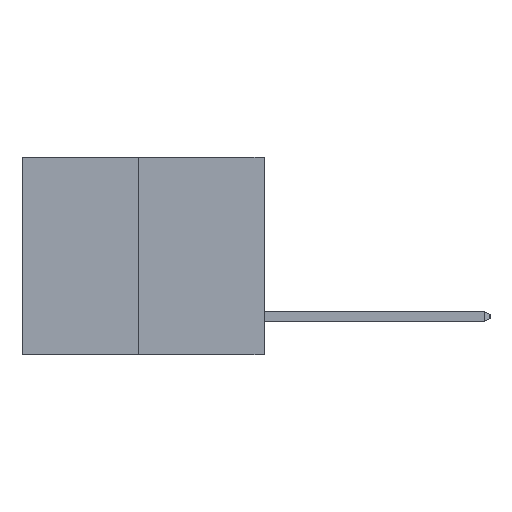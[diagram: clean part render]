
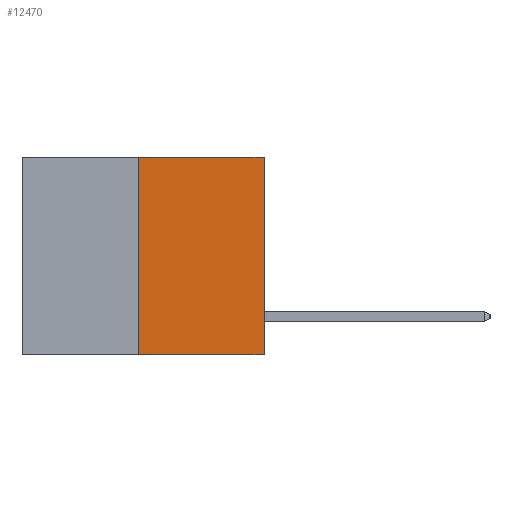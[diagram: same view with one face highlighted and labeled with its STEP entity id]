
A CAD part, left-side view. The second image highlights one B-rep face of the part: STEP entity #12470.
In plain terms, the highlighted planar face has unit normal (-1, 0, 0).
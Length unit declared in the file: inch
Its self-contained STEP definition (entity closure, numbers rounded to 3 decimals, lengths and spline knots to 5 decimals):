
#847 = ORIENTED_EDGE ( 'NONE', *, *, #9209, .F. ) ;
#1456 = DIRECTION ( 'NONE',  ( 0., 0., 1. ) ) ;
#1790 = PLANE ( 'NONE',  #20895 ) ;
#2164 = ORIENTED_EDGE ( 'NONE', *, *, #15549, .T. ) ;
#3511 = VERTEX_POINT ( 'NONE', #18823 ) ;
#3565 = DIRECTION ( 'NONE',  ( 0., 0., -1. ) ) ;
#3786 = DIRECTION ( 'NONE',  ( 1., 0., 0. ) ) ;
#4258 = EDGE_CURVE ( 'NONE', #3511, #21067, #6278, .T. ) ;
#5006 = LINE ( 'NONE', #19514, #7952 ) ;
#5191 = FACE_OUTER_BOUND ( 'NONE', #20338, .T. ) ;
#6278 = LINE ( 'NONE', #20141, #17500 ) ;
#6523 = LINE ( 'NONE', #18433, #20125 ) ;
#7952 = VECTOR ( 'NONE', #9261, 39.37008 ) ;
#8284 = DIRECTION ( 'NONE',  ( 0., 0., 1. ) ) ;
#9209 = EDGE_CURVE ( 'NONE', #15320, #20425, #6523, .T. ) ;
#9261 = DIRECTION ( 'NONE',  ( 0., -1., 0. ) ) ;
#9698 = CARTESIAN_POINT ( 'NONE',  ( 0., 0., 0. ) ) ;
#9887 = EDGE_CURVE ( 'NONE', #20425, #21067, #5006, .T. ) ;
#10288 = LINE ( 'NONE', #18601, #11376 ) ;
#11376 = VECTOR ( 'NONE', #18529, 39.37008 ) ;
#12470 = ADVANCED_FACE ( 'NONE', ( #5191 ), #1790, .F. ) ;
#13652 = ORIENTED_EDGE ( 'NONE', *, *, #4258, .T. ) ;
#14520 = CARTESIAN_POINT ( 'NONE',  ( 0., 0.312, 0. ) ) ;
#15320 = VERTEX_POINT ( 'NONE', #19603 ) ;
#15549 = EDGE_CURVE ( 'NONE', #15320, #3511, #10288, .T. ) ;
#17500 = VECTOR ( 'NONE', #1456, 39.37008 ) ;
#17720 = ORIENTED_EDGE ( 'NONE', *, *, #9887, .F. ) ;
#18433 = CARTESIAN_POINT ( 'NONE',  ( 0., 0.312, -0.49 ) ) ;
#18529 = DIRECTION ( 'NONE',  ( 0., -1., 0. ) ) ;
#18601 = CARTESIAN_POINT ( 'NONE',  ( 0., 0.6, -0.49 ) ) ;
#18823 = CARTESIAN_POINT ( 'NONE',  ( 0., 0., -0.49 ) ) ;
#18998 = CARTESIAN_POINT ( 'NONE',  ( 0., 0.6, 0. ) ) ;
#19514 = CARTESIAN_POINT ( 'NONE',  ( 0., 0.6, 0. ) ) ;
#19603 = CARTESIAN_POINT ( 'NONE',  ( 0., 0.312, -0.49 ) ) ;
#20125 = VECTOR ( 'NONE', #8284, 39.37008 ) ;
#20141 = CARTESIAN_POINT ( 'NONE',  ( 0., 0., 0. ) ) ;
#20338 = EDGE_LOOP ( 'NONE', ( #847, #2164, #13652, #17720 ) ) ;
#20425 = VERTEX_POINT ( 'NONE', #14520 ) ;
#20895 = AXIS2_PLACEMENT_3D ( 'NONE', #18998, #3786, #3565 ) ;
#21067 = VERTEX_POINT ( 'NONE', #9698 ) ;
